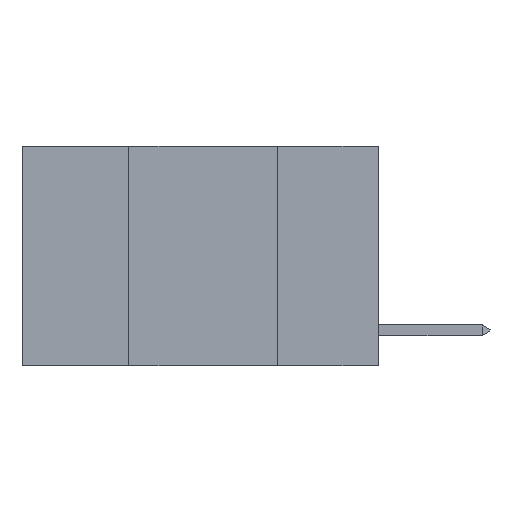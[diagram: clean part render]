
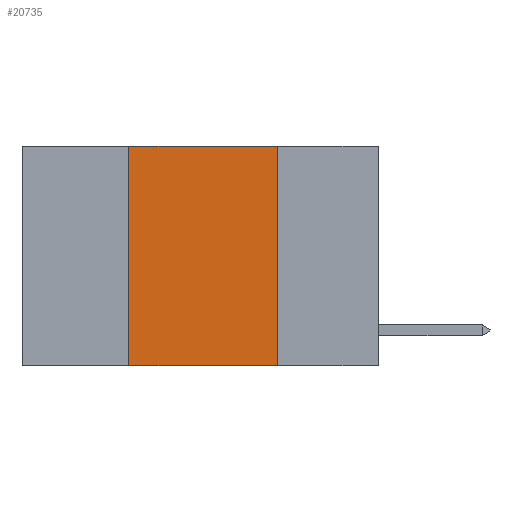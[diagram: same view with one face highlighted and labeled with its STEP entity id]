
A CAD part, left-side view. The second image highlights one B-rep face of the part: STEP entity #20735.
In plain terms, the highlighted planar face has unit normal (-1, 0, 0).
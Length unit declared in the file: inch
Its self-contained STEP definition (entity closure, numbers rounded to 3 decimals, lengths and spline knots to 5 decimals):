
#1163 = CARTESIAN_POINT ( 'NONE',  ( 0., 0.6, -0.37 ) ) ;
#2185 = VERTEX_POINT ( 'NONE', #21258 ) ;
#3644 = VERTEX_POINT ( 'NONE', #21198 ) ;
#3664 = EDGE_CURVE ( 'NONE', #2185, #11105, #4776, .T. ) ;
#3791 = LINE ( 'NONE', #12708, #12594 ) ;
#4776 = LINE ( 'NONE', #1163, #14845 ) ;
#5537 = AXIS2_PLACEMENT_3D ( 'NONE', #21573, #8351, #21333 ) ;
#5826 = CARTESIAN_POINT ( 'NONE',  ( 0., 0.17, -0.37 ) ) ;
#6456 = EDGE_CURVE ( 'NONE', #3644, #11105, #3791, .T. ) ;
#7558 = ORIENTED_EDGE ( 'NONE', *, *, #6456, .F. ) ;
#7568 = EDGE_LOOP ( 'NONE', ( #7558, #10600, #23065, #23638 ) ) ;
#8351 = DIRECTION ( 'NONE',  ( 1., 0., 0. ) ) ;
#10534 = FACE_OUTER_BOUND ( 'NONE', #7568, .T. ) ;
#10600 = ORIENTED_EDGE ( 'NONE', *, *, #20103, .F. ) ;
#10965 = DIRECTION ( 'NONE',  ( 0., -1., 0. ) ) ;
#11105 = VERTEX_POINT ( 'NONE', #5826 ) ;
#12052 = CARTESIAN_POINT ( 'NONE',  ( 0., 0.42, 0. ) ) ;
#12594 = VECTOR ( 'NONE', #20085, 39.37008 ) ;
#12708 = CARTESIAN_POINT ( 'NONE',  ( 0., 0.17, 0. ) ) ;
#13928 = DIRECTION ( 'NONE',  ( 0., -1., 0. ) ) ;
#14845 = VECTOR ( 'NONE', #13928, 39.37008 ) ;
#15343 = LINE ( 'NONE', #19573, #18623 ) ;
#17800 = PLANE ( 'NONE',  #5537 ) ;
#18623 = VECTOR ( 'NONE', #21640, 39.37008 ) ;
#19573 = CARTESIAN_POINT ( 'NONE',  ( 0., 0.42, 0. ) ) ;
#20085 = DIRECTION ( 'NONE',  ( 0., 0., -1. ) ) ;
#20103 = EDGE_CURVE ( 'NONE', #20424, #3644, #20167, .T. ) ;
#20167 = LINE ( 'NONE', #21760, #20547 ) ;
#20424 = VERTEX_POINT ( 'NONE', #12052 ) ;
#20547 = VECTOR ( 'NONE', #10965, 39.37008 ) ;
#20735 = ADVANCED_FACE ( 'NONE', ( #10534 ), #17800, .F. ) ;
#21198 = CARTESIAN_POINT ( 'NONE',  ( 0., 0.17, 0. ) ) ;
#21258 = CARTESIAN_POINT ( 'NONE',  ( 0., 0.42, -0.37 ) ) ;
#21333 = DIRECTION ( 'NONE',  ( 0., 0., -1. ) ) ;
#21573 = CARTESIAN_POINT ( 'NONE',  ( 0., 0.6, 0. ) ) ;
#21640 = DIRECTION ( 'NONE',  ( 0., 0., 1. ) ) ;
#21760 = CARTESIAN_POINT ( 'NONE',  ( 0., 0.6, 0. ) ) ;
#21884 = EDGE_CURVE ( 'NONE', #2185, #20424, #15343, .T. ) ;
#23065 = ORIENTED_EDGE ( 'NONE', *, *, #21884, .F. ) ;
#23638 = ORIENTED_EDGE ( 'NONE', *, *, #3664, .T. ) ;
